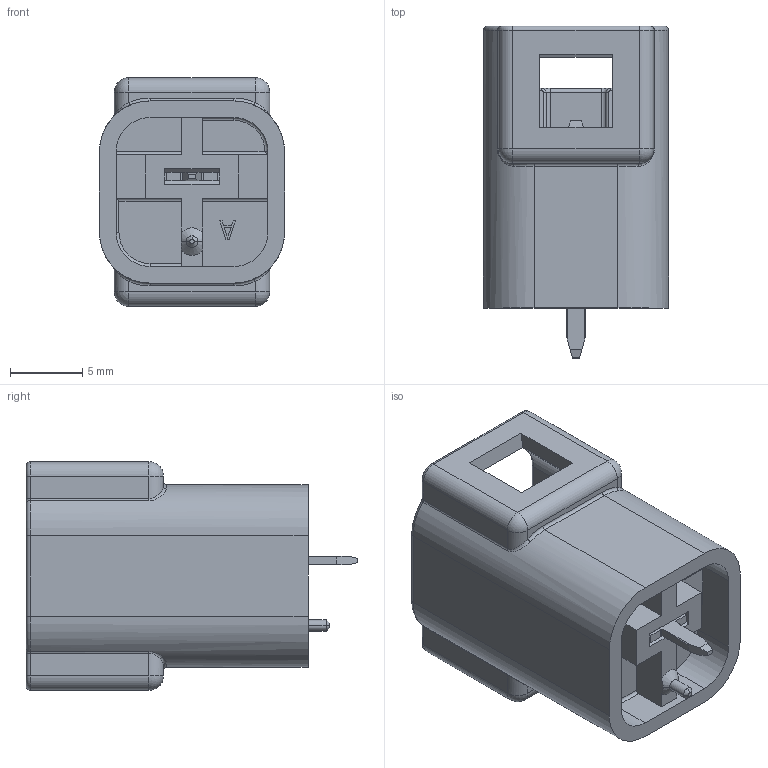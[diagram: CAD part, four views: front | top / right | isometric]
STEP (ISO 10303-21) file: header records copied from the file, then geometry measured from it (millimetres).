
FILE_DESCRIPTION (( 'STEP AP214' ), '1' );
FILE_NAME ('572-001-420-301.STEP', '2020-07-30T16:35:28', ( '' ), ( '' ), 'SwSTEP 2.0', 'SolidWorks 2020', '' );
FILE_SCHEMA (( 'AUTOMOTIVE_DESIGN' ));
Length unit declared in the file: millimetre
Products named in the file (3): 572-001-420-PCB HOUSING_BLUE; 572-001-420-301; 570-420 PCB-TERMINAL-1
Assembly tree (2 placements, depth 2):
  572-001-420-301
    572-001-420-PCB HOUSING_BLUE
    570-420 PCB-TERMINAL-1
Bounding box: 12.8 x 22.95 x 15.8 mm (x, y, z)
Volume: 1297.7 mm3; surface area: 2370.4 mm2
Topology: 2 solids, 2 shells, 305 faces, 777 edges, 475 vertices
Faces by surface type: plane 154, cylinder 90, torus 36, bspline 10, cone 9, sphere 6
Entity records: 9585 total; most frequent: CARTESIAN_POINT 2151, ORIENTED_EDGE 1540, DIRECTION 1534, EDGE_CURVE 770, VECTOR 514, LINE 514, AXIS2_PLACEMENT_3D 510, VERTEX_POINT 474
